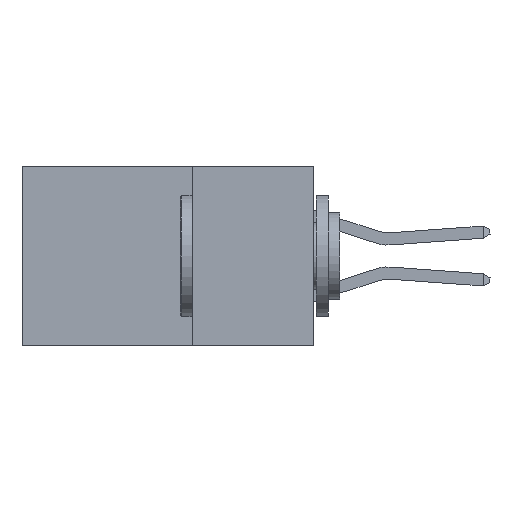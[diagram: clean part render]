
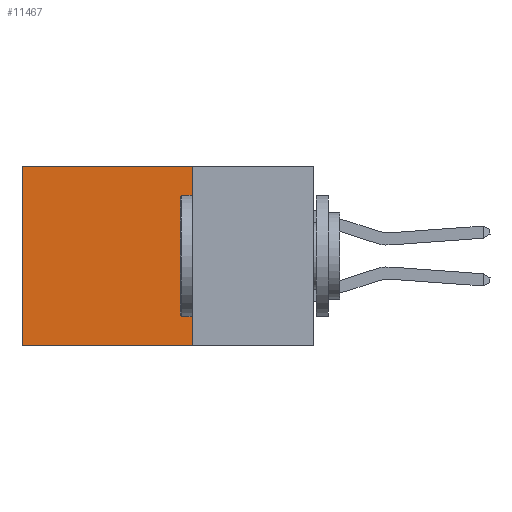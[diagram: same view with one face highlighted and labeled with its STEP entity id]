
A CAD part, left-side view. The second image highlights one B-rep face of the part: STEP entity #11467.
In plain terms, the highlighted planar face has unit normal (-1, 0, 0).
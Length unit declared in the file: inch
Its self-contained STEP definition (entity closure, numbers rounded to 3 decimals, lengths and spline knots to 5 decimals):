
#1022 = ORIENTED_EDGE ( 'NONE', *, *, #2076, .T. ) ;
#1877 = EDGE_LOOP ( 'NONE', ( #1022, #25305, #16915, #19526 ) ) ;
#2040 = LINE ( 'NONE', #26162, #29471 ) ;
#2076 = EDGE_CURVE ( 'NONE', #5729, #6642, #24502, .T. ) ;
#3834 = DIRECTION ( 'NONE',  ( 0., 1., 0. ) ) ;
#4549 = EDGE_CURVE ( 'NONE', #19437, #18740, #2040, .T. ) ;
#5729 = VERTEX_POINT ( 'NONE', #20028 ) ;
#6642 = VERTEX_POINT ( 'NONE', #20502 ) ;
#7875 = LINE ( 'NONE', #31830, #12538 ) ;
#7914 = CARTESIAN_POINT ( 'NONE',  ( 0.2875, 0.25, -0.37 ) ) ;
#8366 = AXIS2_PLACEMENT_3D ( 'NONE', #16469, #26246, #24139 ) ;
#8389 = DIRECTION ( 'NONE',  ( 0., 1., 0. ) ) ;
#8426 = CARTESIAN_POINT ( 'NONE',  ( 0.2875, 0.25, 0. ) ) ;
#8832 = CARTESIAN_POINT ( 'NONE',  ( 0.2875, 0.25, -0.37 ) ) ;
#11467 = ADVANCED_FACE ( 'NONE', ( #16423 ), #31157, .F. ) ;
#12538 = VECTOR ( 'NONE', #8389, 39.37008 ) ;
#13403 = DIRECTION ( 'NONE',  ( 0., 0., -1. ) ) ;
#13927 = EDGE_CURVE ( 'NONE', #19437, #5729, #7875, .T. ) ;
#16423 = FACE_OUTER_BOUND ( 'NONE', #1877, .T. ) ;
#16469 = CARTESIAN_POINT ( 'NONE',  ( 0.2875, 0.25, 0. ) ) ;
#16915 = ORIENTED_EDGE ( 'NONE', *, *, #4549, .F. ) ;
#18338 = LINE ( 'NONE', #8832, #30527 ) ;
#18740 = VERTEX_POINT ( 'NONE', #7914 ) ;
#19437 = VERTEX_POINT ( 'NONE', #8426 ) ;
#19526 = ORIENTED_EDGE ( 'NONE', *, *, #13927, .T. ) ;
#20028 = CARTESIAN_POINT ( 'NONE',  ( 0.2875, 0.6, 0. ) ) ;
#20502 = CARTESIAN_POINT ( 'NONE',  ( 0.2875, 0.6, -0.37 ) ) ;
#20720 = CARTESIAN_POINT ( 'NONE',  ( 0.2875, 0.6, 0. ) ) ;
#24139 = DIRECTION ( 'NONE',  ( 0., 0., -1. ) ) ;
#24502 = LINE ( 'NONE', #20720, #27992 ) ;
#25305 = ORIENTED_EDGE ( 'NONE', *, *, #30247, .F. ) ;
#26162 = CARTESIAN_POINT ( 'NONE',  ( 0.2875, 0.25, 0. ) ) ;
#26246 = DIRECTION ( 'NONE',  ( 1., 0., 0. ) ) ;
#27992 = VECTOR ( 'NONE', #31480, 39.37008 ) ;
#29471 = VECTOR ( 'NONE', #13403, 39.37008 ) ;
#30247 = EDGE_CURVE ( 'NONE', #18740, #6642, #18338, .T. ) ;
#30527 = VECTOR ( 'NONE', #3834, 39.37008 ) ;
#31157 = PLANE ( 'NONE',  #8366 ) ;
#31480 = DIRECTION ( 'NONE',  ( 0., 0., -1. ) ) ;
#31830 = CARTESIAN_POINT ( 'NONE',  ( 0.2875, 0.25, 0. ) ) ;
